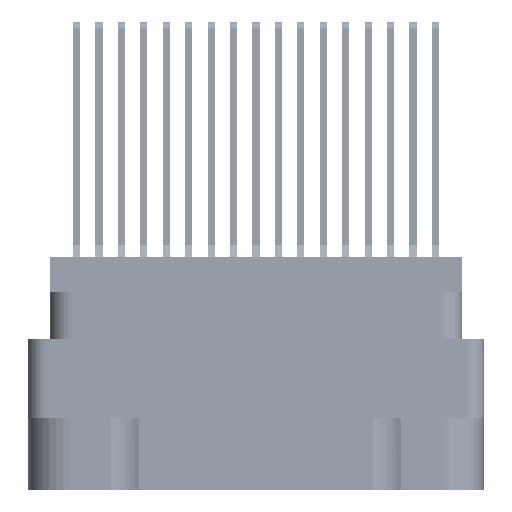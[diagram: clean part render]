
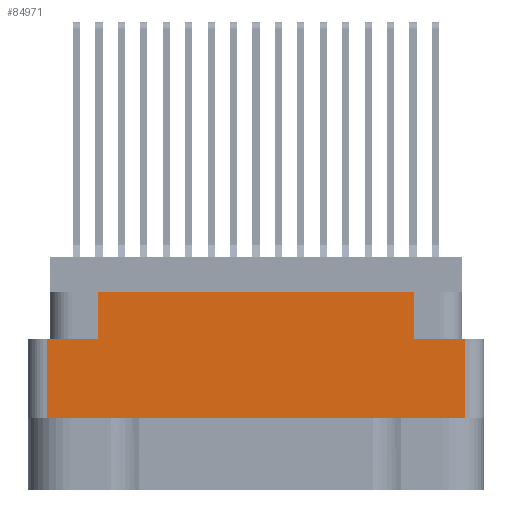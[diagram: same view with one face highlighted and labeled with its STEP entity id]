
A CAD part, left-side view. The second image highlights one B-rep face of the part: STEP entity #84971.
In plain terms, the highlighted planar face has unit normal (-1, 0, 0).
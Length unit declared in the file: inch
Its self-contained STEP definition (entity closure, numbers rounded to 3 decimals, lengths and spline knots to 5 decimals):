
#2172 = LINE ( 'NONE', #28234, #53593 ) ;
#2651 = DIRECTION ( 'NONE',  ( 0., 0., 1. ) ) ;
#2701 = VECTOR ( 'NONE', #37992, 39.37008 ) ;
#5135 = EDGE_CURVE ( 'NONE', #23663, #13321, #15208, .T. ) ;
#6463 = DIRECTION ( 'NONE',  ( 0., 0., 1. ) ) ;
#9933 = EDGE_CURVE ( 'NONE', #46061, #82455, #60378, .T. ) ;
#11558 = ORIENTED_EDGE ( 'NONE', *, *, #72180, .F. ) ;
#11976 = LINE ( 'NONE', #64194, #27705 ) ;
#13321 = VERTEX_POINT ( 'NONE', #54329 ) ;
#13659 = CARTESIAN_POINT ( 'NONE',  ( -1.375, 0., -0.54 ) ) ;
#15208 = LINE ( 'NONE', #80642, #18409 ) ;
#16814 = ORIENTED_EDGE ( 'NONE', *, *, #9933, .T. ) ;
#16898 = CARTESIAN_POINT ( 'NONE',  ( -1.375, 0.5285, -0.117 ) ) ;
#16937 = DIRECTION ( 'NONE',  ( 0., 0., 1. ) ) ;
#18119 = CARTESIAN_POINT ( 'NONE',  ( -1.375, -0.7005, -0.54 ) ) ;
#18409 = VECTOR ( 'NONE', #33195, 39.37008 ) ;
#19209 = ORIENTED_EDGE ( 'NONE', *, *, #62575, .F. ) ;
#20570 = DIRECTION ( 'NONE',  ( 0., -1., 0. ) ) ;
#23663 = VERTEX_POINT ( 'NONE', #16898 ) ;
#26251 = LINE ( 'NONE', #47518, #35688 ) ;
#27705 = VECTOR ( 'NONE', #43987, 39.37008 ) ;
#28234 = CARTESIAN_POINT ( 'NONE',  ( -1.375, 0., -0.274 ) ) ;
#30909 = ORIENTED_EDGE ( 'NONE', *, *, #5135, .F. ) ;
#33195 = DIRECTION ( 'NONE',  ( 0., -1., 0. ) ) ;
#33633 = DIRECTION ( 'NONE',  ( 0., -1., 0. ) ) ;
#35688 = VECTOR ( 'NONE', #6463, 39.37008 ) ;
#37992 = DIRECTION ( 'NONE',  ( 0., 0., 1. ) ) ;
#38679 = CARTESIAN_POINT ( 'NONE',  ( -1.375, -0.7625, -0.78 ) ) ;
#40834 = CARTESIAN_POINT ( 'NONE',  ( -1.375, 0., -0.274 ) ) ;
#41058 = VECTOR ( 'NONE', #2651, 39.37008 ) ;
#43987 = DIRECTION ( 'NONE',  ( 0., 0., -1. ) ) ;
#44247 = LINE ( 'NONE', #40834, #71478 ) ;
#44645 = VECTOR ( 'NONE', #33633, 39.37008 ) ;
#45267 = EDGE_CURVE ( 'NONE', #82455, #73161, #26251, .T. ) ;
#46061 = VERTEX_POINT ( 'NONE', #85976 ) ;
#47518 = CARTESIAN_POINT ( 'NONE',  ( -1.375, -0.7005, -0.78 ) ) ;
#49579 = CARTESIAN_POINT ( 'NONE',  ( -1.375, -0.7005, -0.274 ) ) ;
#52107 = CARTESIAN_POINT ( 'NONE',  ( -1.375, 0.7005, -0.274 ) ) ;
#53593 = VECTOR ( 'NONE', #75455, 39.37008 ) ;
#54329 = CARTESIAN_POINT ( 'NONE',  ( -1.375, -0.5285, -0.117 ) ) ;
#54661 = VERTEX_POINT ( 'NONE', #58429 ) ;
#56892 = CARTESIAN_POINT ( 'NONE',  ( -1.375, -0.5285, -0.274 ) ) ;
#58429 = CARTESIAN_POINT ( 'NONE',  ( -1.375, -0.5285, -0.274 ) ) ;
#58614 = PLANE ( 'NONE',  #73957 ) ;
#60378 = LINE ( 'NONE', #13659, #44645 ) ;
#60405 = FACE_OUTER_BOUND ( 'NONE', #75752, .T. ) ;
#62529 = LINE ( 'NONE', #65499, #2701 ) ;
#62575 = EDGE_CURVE ( 'NONE', #54661, #73161, #44247, .T. ) ;
#62846 = EDGE_CURVE ( 'NONE', #54661, #13321, #83017, .T. ) ;
#63457 = EDGE_CURVE ( 'NONE', #69639, #86416, #2172, .T. ) ;
#64194 = CARTESIAN_POINT ( 'NONE',  ( -1.375, 0.7005, -0.78 ) ) ;
#65499 = CARTESIAN_POINT ( 'NONE',  ( -1.375, 0.5285, -0.274 ) ) ;
#65904 = DIRECTION ( 'NONE',  ( -1., 0., 0. ) ) ;
#69216 = ORIENTED_EDGE ( 'NONE', *, *, #62846, .T. ) ;
#69639 = VERTEX_POINT ( 'NONE', #52107 ) ;
#70163 = ORIENTED_EDGE ( 'NONE', *, *, #63457, .F. ) ;
#71478 = VECTOR ( 'NONE', #20570, 39.37008 ) ;
#72180 = EDGE_CURVE ( 'NONE', #86416, #23663, #62529, .T. ) ;
#73142 = EDGE_CURVE ( 'NONE', #69639, #46061, #11976, .T. ) ;
#73161 = VERTEX_POINT ( 'NONE', #49579 ) ;
#73957 = AXIS2_PLACEMENT_3D ( 'NONE', #38679, #65904, #16937 ) ;
#75455 = DIRECTION ( 'NONE',  ( 0., -1., 0. ) ) ;
#75752 = EDGE_LOOP ( 'NONE', ( #70163, #77335, #16814, #76671, #19209, #69216, #30909, #11558 ) ) ;
#76671 = ORIENTED_EDGE ( 'NONE', *, *, #45267, .T. ) ;
#77335 = ORIENTED_EDGE ( 'NONE', *, *, #73142, .T. ) ;
#79813 = CARTESIAN_POINT ( 'NONE',  ( -1.375, 0.5285, -0.274 ) ) ;
#80642 = CARTESIAN_POINT ( 'NONE',  ( -1.375, 0.7625, -0.117 ) ) ;
#82455 = VERTEX_POINT ( 'NONE', #18119 ) ;
#83017 = LINE ( 'NONE', #56892, #41058 ) ;
#84971 = ADVANCED_FACE ( 'NONE', ( #60405 ), #58614, .T. ) ;
#85976 = CARTESIAN_POINT ( 'NONE',  ( -1.375, 0.7005, -0.54 ) ) ;
#86416 = VERTEX_POINT ( 'NONE', #79813 ) ;
